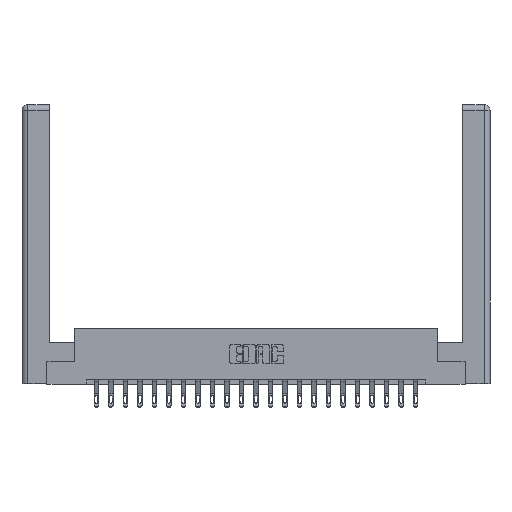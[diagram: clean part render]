
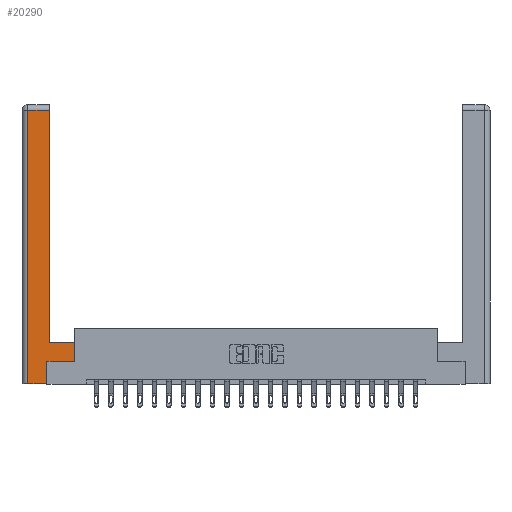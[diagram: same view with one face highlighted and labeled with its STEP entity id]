
A CAD part, top view. The second image highlights one B-rep face of the part: STEP entity #20290.
In plain terms, the highlighted planar face has unit normal (0, 0, 1).
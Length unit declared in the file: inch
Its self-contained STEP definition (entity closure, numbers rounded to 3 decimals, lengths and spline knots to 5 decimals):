
#14 = VECTOR ( 'NONE', #5981, 39.37008 ) ;
#222 = VERTEX_POINT ( 'NONE', #857 ) ;
#857 = CARTESIAN_POINT ( 'NONE',  ( 0.295, 0.45, 0. ) ) ;
#1056 = VECTOR ( 'NONE', #14544, 39.37008 ) ;
#2237 = VERTEX_POINT ( 'NONE', #7517 ) ;
#2306 = CARTESIAN_POINT ( 'NONE',  ( 0.565, 0.45, 0. ) ) ;
#2402 = DIRECTION ( 'NONE',  ( 0., -1., 0. ) ) ;
#2534 = ORIENTED_EDGE ( 'NONE', *, *, #11250, .T. ) ;
#2802 = VERTEX_POINT ( 'NONE', #5998 ) ;
#3613 = VERTEX_POINT ( 'NONE', #19200 ) ;
#4110 = CARTESIAN_POINT ( 'NONE',  ( 0.295, 3., 0. ) ) ;
#5535 = DIRECTION ( 'NONE',  ( -1., 0., 0. ) ) ;
#5817 = LINE ( 'NONE', #8155, #23254 ) ;
#5877 = EDGE_CURVE ( 'NONE', #23260, #3613, #5817, .T. ) ;
#5981 = DIRECTION ( 'NONE',  ( 0., 1., 0. ) ) ;
#5998 = CARTESIAN_POINT ( 'NONE',  ( 0.265, 0., 0. ) ) ;
#6202 = CARTESIAN_POINT ( 'NONE',  ( 0.0615, 0., 0. ) ) ;
#6654 = ORIENTED_EDGE ( 'NONE', *, *, #21884, .T. ) ;
#6673 = VECTOR ( 'NONE', #19910, 39.37008 ) ;
#6701 = ORIENTED_EDGE ( 'NONE', *, *, #14049, .T. ) ;
#6979 = ORIENTED_EDGE ( 'NONE', *, *, #11092, .T. ) ;
#7167 = LINE ( 'NONE', #6202, #20391 ) ;
#7229 = VECTOR ( 'NONE', #21493, 39.37008 ) ;
#7517 = CARTESIAN_POINT ( 'NONE',  ( 0.265, 0.245, 0. ) ) ;
#8155 = CARTESIAN_POINT ( 'NONE',  ( 0.0615, 2.94, 0. ) ) ;
#8507 = ORIENTED_EDGE ( 'NONE', *, *, #17437, .T. ) ;
#9135 = CARTESIAN_POINT ( 'NONE',  ( 0., 0., 0. ) ) ;
#10084 = EDGE_CURVE ( 'NONE', #2237, #20203, #21957, .T. ) ;
#10647 = EDGE_LOOP ( 'NONE', ( #22603, #11853, #6701, #8507, #6654, #10912, #2534, #6979 ) ) ;
#10912 = ORIENTED_EDGE ( 'NONE', *, *, #10084, .T. ) ;
#11040 = CARTESIAN_POINT ( 'NONE',  ( 0.265, 0., 0. ) ) ;
#11092 = EDGE_CURVE ( 'NONE', #21480, #222, #21359, .T. ) ;
#11250 = EDGE_CURVE ( 'NONE', #20203, #21480, #21608, .T. ) ;
#11262 = LINE ( 'NONE', #4110, #14 ) ;
#11853 = ORIENTED_EDGE ( 'NONE', *, *, #5877, .T. ) ;
#11987 = LINE ( 'NONE', #14081, #7229 ) ;
#12195 = VERTEX_POINT ( 'NONE', #14962 ) ;
#12352 = CARTESIAN_POINT ( 'NONE',  ( 0.565, 0.245, 0. ) ) ;
#12666 = PLANE ( 'NONE',  #23219 ) ;
#12723 = VECTOR ( 'NONE', #19813, 39.37008 ) ;
#13759 = VECTOR ( 'NONE', #15751, 39.37008 ) ;
#14049 = EDGE_CURVE ( 'NONE', #3613, #12195, #7167, .T. ) ;
#14081 = CARTESIAN_POINT ( 'NONE',  ( 0.265, 0.245, 0. ) ) ;
#14109 = CARTESIAN_POINT ( 'NONE',  ( 0.565, 0.245, 0. ) ) ;
#14352 = FACE_OUTER_BOUND ( 'NONE', #10647, .T. ) ;
#14544 = DIRECTION ( 'NONE',  ( 0., 1., 0. ) ) ;
#14962 = CARTESIAN_POINT ( 'NONE',  ( 0.0615, 0., 0. ) ) ;
#15751 = DIRECTION ( 'NONE',  ( 1., 0., 0. ) ) ;
#16306 = DIRECTION ( 'NONE',  ( 0., 0., -1. ) ) ;
#17437 = EDGE_CURVE ( 'NONE', #12195, #2802, #17535, .T. ) ;
#17535 = LINE ( 'NONE', #11040, #12723 ) ;
#18221 = EDGE_CURVE ( 'NONE', #222, #23260, #11262, .T. ) ;
#19200 = CARTESIAN_POINT ( 'NONE',  ( 0.0615, 2.94, 0. ) ) ;
#19813 = DIRECTION ( 'NONE',  ( 1., 0., 0. ) ) ;
#19910 = DIRECTION ( 'NONE',  ( -1., 0., 0. ) ) ;
#19917 = CARTESIAN_POINT ( 'NONE',  ( 0.565, 0.45, 0. ) ) ;
#19983 = CARTESIAN_POINT ( 'NONE',  ( 0.295, 0.45, 0. ) ) ;
#20203 = VERTEX_POINT ( 'NONE', #14109 ) ;
#20290 = ADVANCED_FACE ( 'NONE', ( #14352 ), #12666, .F. ) ;
#20391 = VECTOR ( 'NONE', #2402, 39.37008 ) ;
#20614 = DIRECTION ( 'NONE',  ( -1., 0., 0. ) ) ;
#21359 = LINE ( 'NONE', #19983, #6673 ) ;
#21480 = VERTEX_POINT ( 'NONE', #2306 ) ;
#21493 = DIRECTION ( 'NONE',  ( 0., 1., 0. ) ) ;
#21608 = LINE ( 'NONE', #19917, #1056 ) ;
#21884 = EDGE_CURVE ( 'NONE', #2802, #2237, #11987, .T. ) ;
#21957 = LINE ( 'NONE', #12352, #13759 ) ;
#22603 = ORIENTED_EDGE ( 'NONE', *, *, #18221, .T. ) ;
#23007 = CARTESIAN_POINT ( 'NONE',  ( 0.295, 2.94, 0. ) ) ;
#23219 = AXIS2_PLACEMENT_3D ( 'NONE', #9135, #16306, #5535 ) ;
#23254 = VECTOR ( 'NONE', #20614, 39.37008 ) ;
#23260 = VERTEX_POINT ( 'NONE', #23007 ) ;
